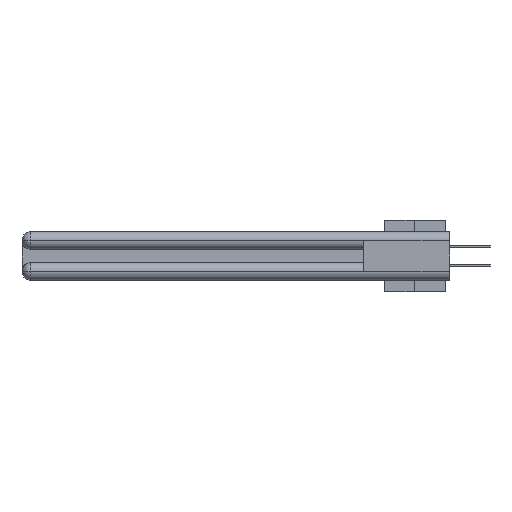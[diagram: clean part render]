
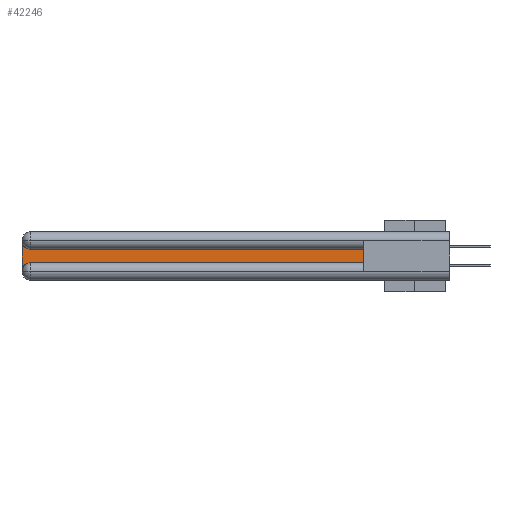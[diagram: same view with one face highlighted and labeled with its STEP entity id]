
A CAD part, left-side view. The second image highlights one B-rep face of the part: STEP entity #42246.
In plain terms, the highlighted planar face has unit normal (-1, 0, 0).
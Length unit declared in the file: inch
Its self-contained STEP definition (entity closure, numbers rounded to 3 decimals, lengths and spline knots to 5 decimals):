
#222 = ORIENTED_EDGE ( 'NONE', *, *, #1990, .T. ) ;
#443 = DIRECTION ( 'NONE',  ( 0., 0., -1. ) ) ;
#1309 = CARTESIAN_POINT ( 'NONE',  ( 0.075, 3., -0.2175 ) ) ;
#1990 = EDGE_CURVE ( 'NONE', #4531, #26484, #4209, .T. ) ;
#2037 = CARTESIAN_POINT ( 'NONE',  ( 0.075, 0.6, -0.2175 ) ) ;
#2606 = EDGE_CURVE ( 'NONE', #37515, #4531, #43171, .T. ) ;
#3763 = ORIENTED_EDGE ( 'NONE', *, *, #14964, .T. ) ;
#4209 = LINE ( 'NONE', #9689, #41675 ) ;
#4531 = VERTEX_POINT ( 'NONE', #23887 ) ;
#4674 = DIRECTION ( 'NONE',  ( 1., 0., 0. ) ) ;
#9689 = CARTESIAN_POINT ( 'NONE',  ( 0.075, 0.6, -0.1225 ) ) ;
#10966 = AXIS2_PLACEMENT_3D ( 'NONE', #43809, #13352, #26970 ) ;
#11844 = ORIENTED_EDGE ( 'NONE', *, *, #24922, .T. ) ;
#12172 = VECTOR ( 'NONE', #27863, 39.37008 ) ;
#13208 = PLANE ( 'NONE',  #10966 ) ;
#13352 = DIRECTION ( 'NONE',  ( 1., 0., 0. ) ) ;
#14193 = CARTESIAN_POINT ( 'NONE',  ( 0.075, 0.6, -0.2175 ) ) ;
#14964 = EDGE_CURVE ( 'NONE', #26756, #16275, #30270, .T. ) ;
#15107 = CARTESIAN_POINT ( 'NONE',  ( 0.075, 3., -0.0625 ) ) ;
#16046 = EDGE_LOOP ( 'NONE', ( #222, #11844, #22313, #3763, #24845, #41226 ) ) ;
#16275 = VERTEX_POINT ( 'NONE', #42385 ) ;
#17117 = VECTOR ( 'NONE', #39912, 39.37008 ) ;
#17734 = CARTESIAN_POINT ( 'NONE',  ( 0.075, 2.94, -0.1225 ) ) ;
#20294 = LINE ( 'NONE', #2037, #17117 ) ;
#20684 = VECTOR ( 'NONE', #28436, 39.37008 ) ;
#20700 = VERTEX_POINT ( 'NONE', #15107 ) ;
#22313 = ORIENTED_EDGE ( 'NONE', *, *, #31730, .T. ) ;
#22585 = AXIS2_PLACEMENT_3D ( 'NONE', #32367, #4674, #25327 ) ;
#23887 = CARTESIAN_POINT ( 'NONE',  ( 0.075, 0.6, -0.1225 ) ) ;
#24845 = ORIENTED_EDGE ( 'NONE', *, *, #40521, .T. ) ;
#24922 = EDGE_CURVE ( 'NONE', #26484, #20700, #28626, .T. ) ;
#25327 = DIRECTION ( 'NONE',  ( 0., 0., -1. ) ) ;
#26484 = VERTEX_POINT ( 'NONE', #17734 ) ;
#26756 = VERTEX_POINT ( 'NONE', #42897 ) ;
#26970 = DIRECTION ( 'NONE',  ( 0., 0., -1. ) ) ;
#27526 = DIRECTION ( 'NONE',  ( 1., 0., 0. ) ) ;
#27863 = DIRECTION ( 'NONE',  ( 0., 0., 1. ) ) ;
#28436 = DIRECTION ( 'NONE',  ( 0., 0., -1. ) ) ;
#28626 = CIRCLE ( 'NONE', #22585, 0.06 ) ;
#30270 = CIRCLE ( 'NONE', #36958, 0.06 ) ;
#30837 = CARTESIAN_POINT ( 'NONE',  ( 0.075, 2.94, -0.2775 ) ) ;
#31730 = EDGE_CURVE ( 'NONE', #20700, #26756, #42624, .T. ) ;
#32367 = CARTESIAN_POINT ( 'NONE',  ( 0.075, 2.94, -0.0625 ) ) ;
#34631 = CARTESIAN_POINT ( 'NONE',  ( 0.075, 0.6, -0.2175 ) ) ;
#36030 = FACE_OUTER_BOUND ( 'NONE', #16046, .T. ) ;
#36958 = AXIS2_PLACEMENT_3D ( 'NONE', #30837, #27526, #443 ) ;
#37515 = VERTEX_POINT ( 'NONE', #14193 ) ;
#39912 = DIRECTION ( 'NONE',  ( 0., -1., 0. ) ) ;
#40521 = EDGE_CURVE ( 'NONE', #16275, #37515, #20294, .T. ) ;
#41226 = ORIENTED_EDGE ( 'NONE', *, *, #2606, .T. ) ;
#41675 = VECTOR ( 'NONE', #44015, 39.37008 ) ;
#42246 = ADVANCED_FACE ( 'NONE', ( #36030 ), #13208, .F. ) ;
#42385 = CARTESIAN_POINT ( 'NONE',  ( 0.075, 2.94, -0.2175 ) ) ;
#42624 = LINE ( 'NONE', #1309, #20684 ) ;
#42897 = CARTESIAN_POINT ( 'NONE',  ( 0.075, 3., -0.2775 ) ) ;
#43171 = LINE ( 'NONE', #34631, #12172 ) ;
#43809 = CARTESIAN_POINT ( 'NONE',  ( 0.075, 3., -0.1225 ) ) ;
#44015 = DIRECTION ( 'NONE',  ( 0., 1., 0. ) ) ;
